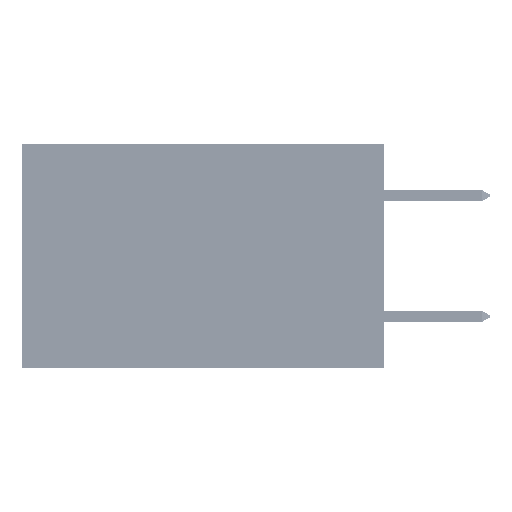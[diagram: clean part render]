
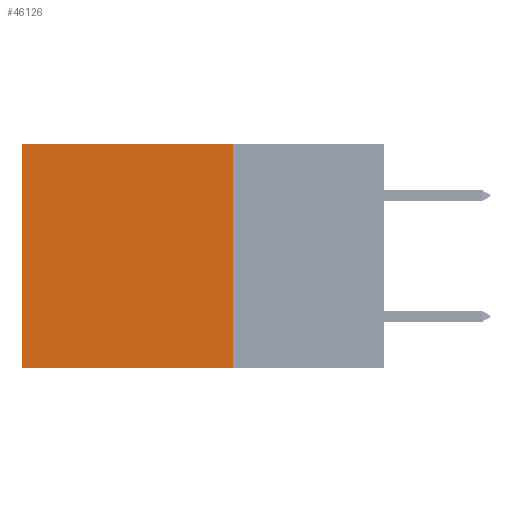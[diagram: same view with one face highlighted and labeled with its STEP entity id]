
A CAD part, left-side view. The second image highlights one B-rep face of the part: STEP entity #46126.
In plain terms, the highlighted planar face has unit normal (-1, 0, 0).
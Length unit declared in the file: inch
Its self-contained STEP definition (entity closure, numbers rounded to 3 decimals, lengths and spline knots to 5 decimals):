
#567 = DIRECTION ( 'NONE',  ( 0., 1., 0. ) ) ;
#3229 = EDGE_CURVE ( 'NONE', #21665, #22025, #17145, .T. ) ;
#3876 = DIRECTION ( 'NONE',  ( 1., 0., 0. ) ) ;
#7100 = VECTOR ( 'NONE', #37271, 39.37008 ) ;
#9852 = AXIS2_PLACEMENT_3D ( 'NONE', #11133, #3876, #33490 ) ;
#11133 = CARTESIAN_POINT ( 'NONE',  ( 0.2875, 0.25, 0. ) ) ;
#11693 = CARTESIAN_POINT ( 'NONE',  ( 0.2875, 0.25, -0.37 ) ) ;
#11801 = EDGE_CURVE ( 'NONE', #39824, #21665, #13918, .T. ) ;
#13668 = ORIENTED_EDGE ( 'NONE', *, *, #39186, .F. ) ;
#13918 = LINE ( 'NONE', #40611, #21368 ) ;
#13950 = ORIENTED_EDGE ( 'NONE', *, *, #3229, .T. ) ;
#15994 = VECTOR ( 'NONE', #39100, 39.37008 ) ;
#16852 = LINE ( 'NONE', #11693, #7100 ) ;
#17145 = LINE ( 'NONE', #24051, #15994 ) ;
#18471 = PLANE ( 'NONE',  #9852 ) ;
#19787 = EDGE_CURVE ( 'NONE', #35308, #22025, #16852, .T. ) ;
#21368 = VECTOR ( 'NONE', #567, 39.37008 ) ;
#21665 = VERTEX_POINT ( 'NONE', #25202 ) ;
#22025 = VERTEX_POINT ( 'NONE', #22637 ) ;
#22637 = CARTESIAN_POINT ( 'NONE',  ( 0.2875, 0.6, -0.37 ) ) ;
#23433 = LINE ( 'NONE', #46517, #38931 ) ;
#24051 = CARTESIAN_POINT ( 'NONE',  ( 0.2875, 0.6, 0. ) ) ;
#25202 = CARTESIAN_POINT ( 'NONE',  ( 0.2875, 0.6, 0. ) ) ;
#28638 = EDGE_LOOP ( 'NONE', ( #13950, #42620, #13668, #40388 ) ) ;
#33490 = DIRECTION ( 'NONE',  ( 0., 0., -1. ) ) ;
#35308 = VERTEX_POINT ( 'NONE', #46677 ) ;
#36184 = CARTESIAN_POINT ( 'NONE',  ( 0.2875, 0.25, 0. ) ) ;
#37271 = DIRECTION ( 'NONE',  ( 0., 1., 0. ) ) ;
#38931 = VECTOR ( 'NONE', #39489, 39.37008 ) ;
#39100 = DIRECTION ( 'NONE',  ( 0., 0., -1. ) ) ;
#39186 = EDGE_CURVE ( 'NONE', #39824, #35308, #23433, .T. ) ;
#39489 = DIRECTION ( 'NONE',  ( 0., 0., -1. ) ) ;
#39824 = VERTEX_POINT ( 'NONE', #36184 ) ;
#40388 = ORIENTED_EDGE ( 'NONE', *, *, #11801, .T. ) ;
#40611 = CARTESIAN_POINT ( 'NONE',  ( 0.2875, 0.25, 0. ) ) ;
#41518 = FACE_OUTER_BOUND ( 'NONE', #28638, .T. ) ;
#42620 = ORIENTED_EDGE ( 'NONE', *, *, #19787, .F. ) ;
#46126 = ADVANCED_FACE ( 'NONE', ( #41518 ), #18471, .F. ) ;
#46517 = CARTESIAN_POINT ( 'NONE',  ( 0.2875, 0.25, 0. ) ) ;
#46677 = CARTESIAN_POINT ( 'NONE',  ( 0.2875, 0.25, -0.37 ) ) ;
